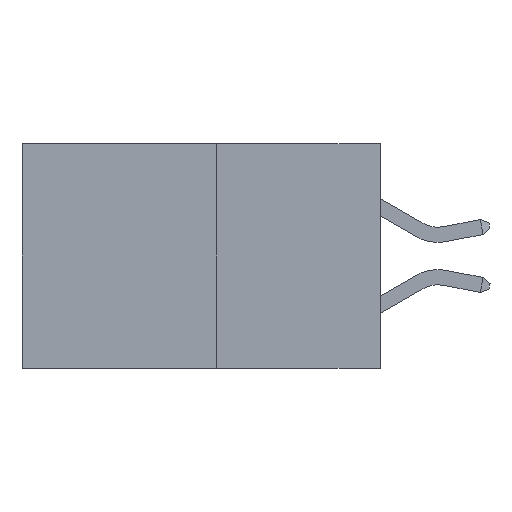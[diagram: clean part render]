
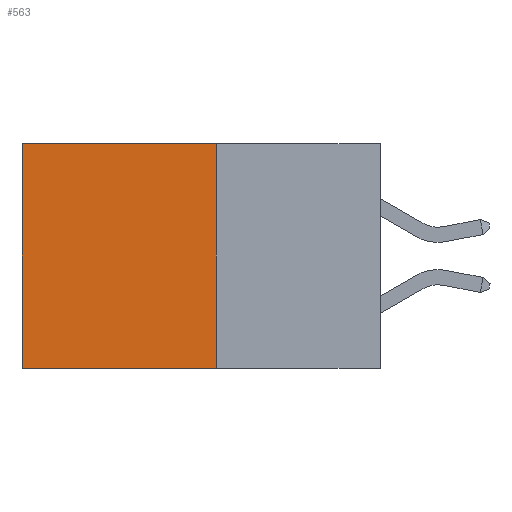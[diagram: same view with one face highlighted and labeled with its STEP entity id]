
A CAD part, left-side view. The second image highlights one B-rep face of the part: STEP entity #563.
In plain terms, the highlighted planar face has unit normal (-1, 0, 0).
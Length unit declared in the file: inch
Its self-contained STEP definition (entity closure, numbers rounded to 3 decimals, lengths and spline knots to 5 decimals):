
#394 = VERTEX_POINT ( 'NONE', #8008 ) ;
#563 = ADVANCED_FACE ( 'NONE', ( #1260 ), #2788, .F. ) ;
#711 = LINE ( 'NONE', #8513, #5396 ) ;
#1260 = FACE_OUTER_BOUND ( 'NONE', #6128, .T. ) ;
#1466 = EDGE_CURVE ( 'NONE', #5766, #3303, #711, .T. ) ;
#1922 = EDGE_CURVE ( 'NONE', #394, #5766, #8860, .T. ) ;
#1954 = CARTESIAN_POINT ( 'NONE',  ( 0.277, 0.59, -0.37 ) ) ;
#2257 = CARTESIAN_POINT ( 'NONE',  ( 0.277, 0.27, -0.37 ) ) ;
#2670 = CARTESIAN_POINT ( 'NONE',  ( 0.277, 0.27, -0.37 ) ) ;
#2732 = VECTOR ( 'NONE', #3376, 39.37008 ) ;
#2788 = PLANE ( 'NONE',  #8880 ) ;
#2930 = DIRECTION ( 'NONE',  ( 0., 0., -1. ) ) ;
#3070 = LINE ( 'NONE', #9079, #7029 ) ;
#3303 = VERTEX_POINT ( 'NONE', #1954 ) ;
#3376 = DIRECTION ( 'NONE',  ( 0., 0., -1. ) ) ;
#4546 = EDGE_CURVE ( 'NONE', #4930, #3303, #5366, .T. ) ;
#4930 = VERTEX_POINT ( 'NONE', #8796 ) ;
#5123 = EDGE_CURVE ( 'NONE', #394, #4930, #3070, .T. ) ;
#5366 = LINE ( 'NONE', #9302, #8931 ) ;
#5396 = VECTOR ( 'NONE', #8502, 39.37008 ) ;
#5461 = ORIENTED_EDGE ( 'NONE', *, *, #4546, .T. ) ;
#5766 = VERTEX_POINT ( 'NONE', #2257 ) ;
#5959 = CARTESIAN_POINT ( 'NONE',  ( 0.277, 0.27, -0.37 ) ) ;
#6128 = EDGE_LOOP ( 'NONE', ( #5461, #9510, #9944, #9672 ) ) ;
#7029 = VECTOR ( 'NONE', #9706, 39.37008 ) ;
#7246 = DIRECTION ( 'NONE',  ( 1., 0., 0. ) ) ;
#8008 = CARTESIAN_POINT ( 'NONE',  ( 0.277, 0.27, 0. ) ) ;
#8502 = DIRECTION ( 'NONE',  ( 0., 1., 0. ) ) ;
#8513 = CARTESIAN_POINT ( 'NONE',  ( 0.277, 0.27, -0.37 ) ) ;
#8796 = CARTESIAN_POINT ( 'NONE',  ( 0.277, 0.59, 0. ) ) ;
#8860 = LINE ( 'NONE', #2670, #2732 ) ;
#8880 = AXIS2_PLACEMENT_3D ( 'NONE', #5959, #7246, #2930 ) ;
#8931 = VECTOR ( 'NONE', #9688, 39.37008 ) ;
#9079 = CARTESIAN_POINT ( 'NONE',  ( 0.277, 0.27, 0. ) ) ;
#9302 = CARTESIAN_POINT ( 'NONE',  ( 0.277, 0.59, -0.37 ) ) ;
#9510 = ORIENTED_EDGE ( 'NONE', *, *, #1466, .F. ) ;
#9672 = ORIENTED_EDGE ( 'NONE', *, *, #5123, .T. ) ;
#9688 = DIRECTION ( 'NONE',  ( 0., 0., -1. ) ) ;
#9706 = DIRECTION ( 'NONE',  ( 0., 1., 0. ) ) ;
#9944 = ORIENTED_EDGE ( 'NONE', *, *, #1922, .F. ) ;
